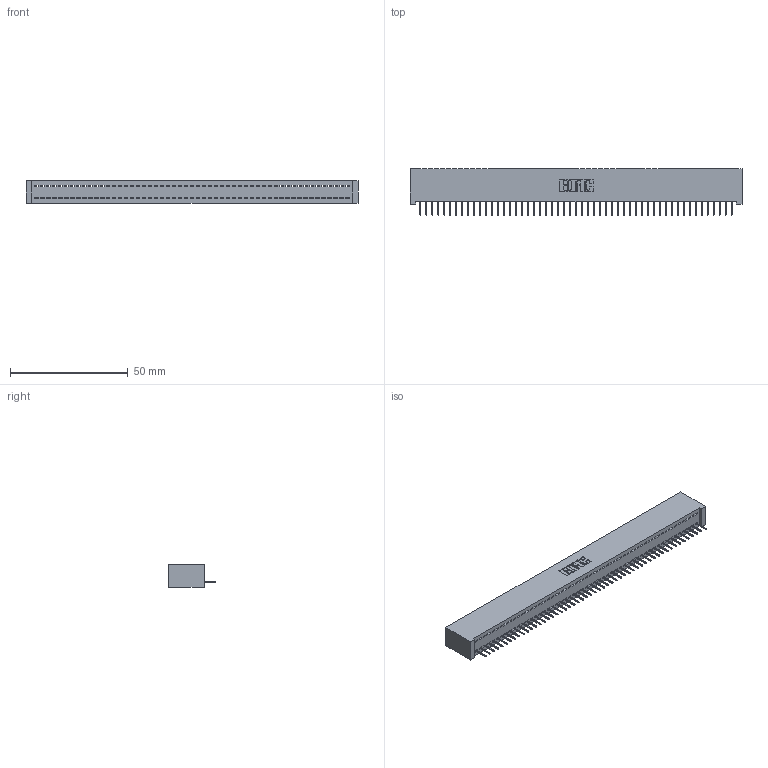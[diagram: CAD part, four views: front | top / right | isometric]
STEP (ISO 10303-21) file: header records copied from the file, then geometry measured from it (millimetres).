
FILE_DESCRIPTION (( 'STEP AP203' ), '1' );
FILE_NAME ('392-053-524-101.STEP', '2019-10-08T13:07:32', ( '' ), ( '' ), 'SwSTEP 2.0', 'SolidWorks 2016', '' );
FILE_SCHEMA (( 'CONFIG_CONTROL_DESIGN' ));
Length unit declared in the file: inch
Products named in the file (3): 342 Part_Lugless; 345-292-001_345-293-124; 392-053-524-101
Assembly tree (54 placements, depth 2):
  392-053-524-101
    342 Part_Lugless
    345-292-001_345-293-124  x53
Bounding box: 140.87 x 19.69 x 9.4 mm (x, y, z)
Volume: 12591.5 mm3; surface area: 18368.4 mm2
Topology: 54 solids, 54 shells, 3388 faces, 9815 edges, 6330 vertices
Faces by surface type: plane 2606, cylinder 782
Entity records: 30643 total; most frequent: CARTESIAN_POINT 5289, ORIENTED_EDGE 5278, DIRECTION 4433, EDGE_CURVE 2639, LINE 2523, VECTOR 2523, VERTEX_POINT 1754, AXIS2_PLACEMENT_3D 955
